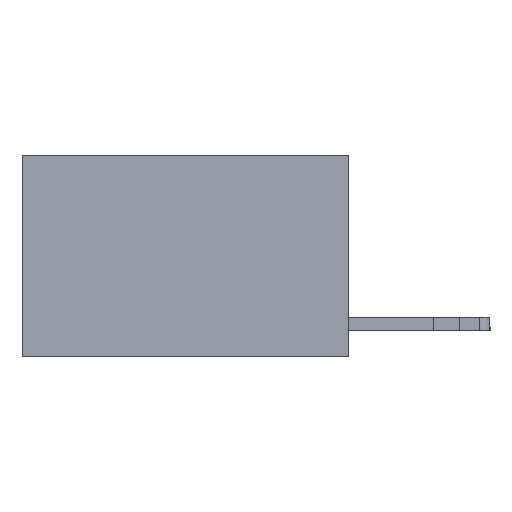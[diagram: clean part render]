
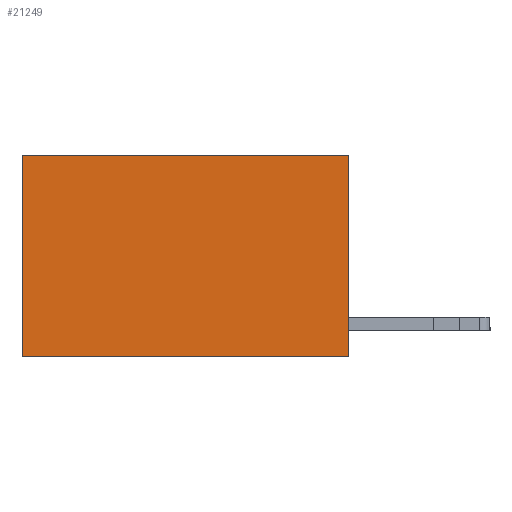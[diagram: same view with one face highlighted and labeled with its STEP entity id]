
A CAD part, left-side view. The second image highlights one B-rep face of the part: STEP entity #21249.
In plain terms, the highlighted planar face has unit normal (-1, 0, 0).
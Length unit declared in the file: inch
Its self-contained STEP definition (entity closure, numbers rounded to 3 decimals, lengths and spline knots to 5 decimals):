
#1337 = DIRECTION ( 'NONE',  ( 0., 1., 0. ) ) ;
#1557 = DIRECTION ( 'NONE',  ( 0., 0., -1. ) ) ;
#1615 = VECTOR ( 'NONE', #10845, 39.37008 ) ;
#2721 = VERTEX_POINT ( 'NONE', #10703 ) ;
#3868 = EDGE_CURVE ( 'NONE', #14007, #27023, #23443, .T. ) ;
#6423 = CARTESIAN_POINT ( 'NONE',  ( 0.2625, 0., -0.37 ) ) ;
#8097 = EDGE_CURVE ( 'NONE', #27023, #2721, #18931, .T. ) ;
#8300 = DIRECTION ( 'NONE',  ( 0., 0., -1. ) ) ;
#8608 = CARTESIAN_POINT ( 'NONE',  ( 0.2625, 0.6, 0. ) ) ;
#9472 = FACE_OUTER_BOUND ( 'NONE', #26154, .T. ) ;
#9900 = VERTEX_POINT ( 'NONE', #6423 ) ;
#9971 = CARTESIAN_POINT ( 'NONE',  ( 0.2625, 0., 0. ) ) ;
#10695 = ORIENTED_EDGE ( 'NONE', *, *, #15781, .F. ) ;
#10703 = CARTESIAN_POINT ( 'NONE',  ( 0.2625, 0.6, -0.37 ) ) ;
#10716 = CARTESIAN_POINT ( 'NONE',  ( 0.2625, 0., 0. ) ) ;
#10845 = DIRECTION ( 'NONE',  ( 0., 1., 0. ) ) ;
#13801 = CARTESIAN_POINT ( 'NONE',  ( 0.2625, 0., 0. ) ) ;
#14007 = VERTEX_POINT ( 'NONE', #24559 ) ;
#15781 = EDGE_CURVE ( 'NONE', #14007, #9900, #20736, .T. ) ;
#16852 = CARTESIAN_POINT ( 'NONE',  ( 0.2625, 0., -0.37 ) ) ;
#18001 = DIRECTION ( 'NONE',  ( 0., 0., -1. ) ) ;
#18931 = LINE ( 'NONE', #26837, #20940 ) ;
#19924 = VECTOR ( 'NONE', #1557, 39.37008 ) ;
#20181 = ORIENTED_EDGE ( 'NONE', *, *, #8097, .T. ) ;
#20658 = LINE ( 'NONE', #16852, #24997 ) ;
#20736 = LINE ( 'NONE', #9971, #19924 ) ;
#20940 = VECTOR ( 'NONE', #8300, 39.37008 ) ;
#21249 = ADVANCED_FACE ( 'NONE', ( #9472 ), #22326, .F. ) ;
#21409 = EDGE_CURVE ( 'NONE', #9900, #2721, #20658, .T. ) ;
#22326 = PLANE ( 'NONE',  #23635 ) ;
#23204 = ORIENTED_EDGE ( 'NONE', *, *, #3868, .T. ) ;
#23443 = LINE ( 'NONE', #10716, #1615 ) ;
#23635 = AXIS2_PLACEMENT_3D ( 'NONE', #13801, #24711, #18001 ) ;
#24559 = CARTESIAN_POINT ( 'NONE',  ( 0.2625, 0., 0. ) ) ;
#24711 = DIRECTION ( 'NONE',  ( 1., 0., 0. ) ) ;
#24997 = VECTOR ( 'NONE', #1337, 39.37008 ) ;
#26154 = EDGE_LOOP ( 'NONE', ( #20181, #27448, #10695, #23204 ) ) ;
#26837 = CARTESIAN_POINT ( 'NONE',  ( 0.2625, 0.6, 0. ) ) ;
#27023 = VERTEX_POINT ( 'NONE', #8608 ) ;
#27448 = ORIENTED_EDGE ( 'NONE', *, *, #21409, .F. ) ;
